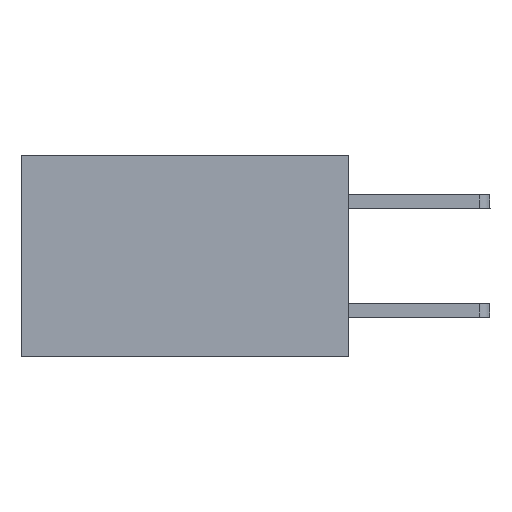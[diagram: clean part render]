
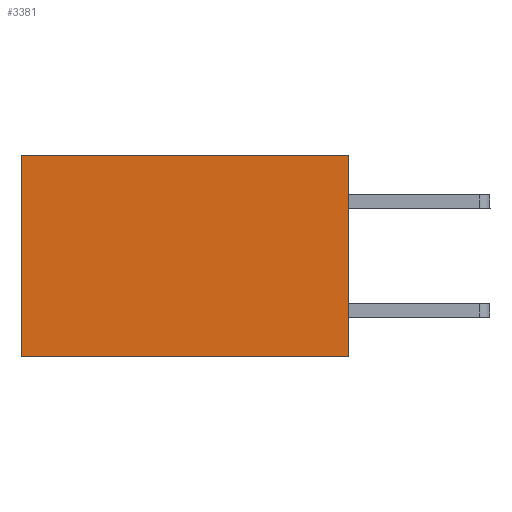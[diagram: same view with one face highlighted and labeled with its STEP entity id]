
A CAD part, left-side view. The second image highlights one B-rep face of the part: STEP entity #3381.
In plain terms, the highlighted planar face has unit normal (-1, 0, 0).
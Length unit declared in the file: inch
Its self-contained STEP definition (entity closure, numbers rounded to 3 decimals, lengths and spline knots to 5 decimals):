
#56 = DIRECTION ( 'NONE',  ( 0., 0., -1. ) ) ;
#590 = CARTESIAN_POINT ( 'NONE',  ( 0.2615, 0., -0.37 ) ) ;
#714 = EDGE_CURVE ( 'NONE', #5174, #9010, #3680, .T. ) ;
#870 = AXIS2_PLACEMENT_3D ( 'NONE', #920, #3686, #56 ) ;
#920 = CARTESIAN_POINT ( 'NONE',  ( 0.2615, 0., -0.37 ) ) ;
#1873 = CARTESIAN_POINT ( 'NONE',  ( 0.2615, 0., 0. ) ) ;
#1982 = CARTESIAN_POINT ( 'NONE',  ( 0.2615, 0.6, 0. ) ) ;
#2569 = DIRECTION ( 'NONE',  ( 0., 0., -1. ) ) ;
#2591 = ORIENTED_EDGE ( 'NONE', *, *, #9687, .F. ) ;
#2744 = DIRECTION ( 'NONE',  ( 0., 0., -1. ) ) ;
#3200 = VECTOR ( 'NONE', #2569, 39.37008 ) ;
#3269 = CARTESIAN_POINT ( 'NONE',  ( 0.2615, 0., 0. ) ) ;
#3381 = ADVANCED_FACE ( 'NONE', ( #4541 ), #4418, .F. ) ;
#3680 = LINE ( 'NONE', #9716, #6119 ) ;
#3686 = DIRECTION ( 'NONE',  ( 1., 0., 0. ) ) ;
#4151 = EDGE_LOOP ( 'NONE', ( #6634, #9420, #2591, #9205 ) ) ;
#4418 = PLANE ( 'NONE',  #870 ) ;
#4541 = FACE_OUTER_BOUND ( 'NONE', #4151, .T. ) ;
#5046 = LINE ( 'NONE', #8577, #3200 ) ;
#5174 = VERTEX_POINT ( 'NONE', #1982 ) ;
#5647 = CARTESIAN_POINT ( 'NONE',  ( 0.2615, 0.6, -0.37 ) ) ;
#5904 = VECTOR ( 'NONE', #9283, 39.37008 ) ;
#5911 = CARTESIAN_POINT ( 'NONE',  ( 0.2615, 0., -0.37 ) ) ;
#6119 = VECTOR ( 'NONE', #2744, 39.37008 ) ;
#6625 = EDGE_CURVE ( 'NONE', #6680, #9010, #9171, .T. ) ;
#6634 = ORIENTED_EDGE ( 'NONE', *, *, #714, .T. ) ;
#6680 = VERTEX_POINT ( 'NONE', #5911 ) ;
#6746 = DIRECTION ( 'NONE',  ( 0., 1., 0. ) ) ;
#7801 = EDGE_CURVE ( 'NONE', #10296, #5174, #11071, .T. ) ;
#8577 = CARTESIAN_POINT ( 'NONE',  ( 0.2615, 0., -0.37 ) ) ;
#9010 = VERTEX_POINT ( 'NONE', #5647 ) ;
#9171 = LINE ( 'NONE', #590, #5904 ) ;
#9205 = ORIENTED_EDGE ( 'NONE', *, *, #7801, .T. ) ;
#9283 = DIRECTION ( 'NONE',  ( 0., 1., 0. ) ) ;
#9420 = ORIENTED_EDGE ( 'NONE', *, *, #6625, .F. ) ;
#9570 = VECTOR ( 'NONE', #6746, 39.37008 ) ;
#9687 = EDGE_CURVE ( 'NONE', #10296, #6680, #5046, .T. ) ;
#9716 = CARTESIAN_POINT ( 'NONE',  ( 0.2615, 0.6, -0.37 ) ) ;
#10296 = VERTEX_POINT ( 'NONE', #1873 ) ;
#11071 = LINE ( 'NONE', #3269, #9570 ) ;
